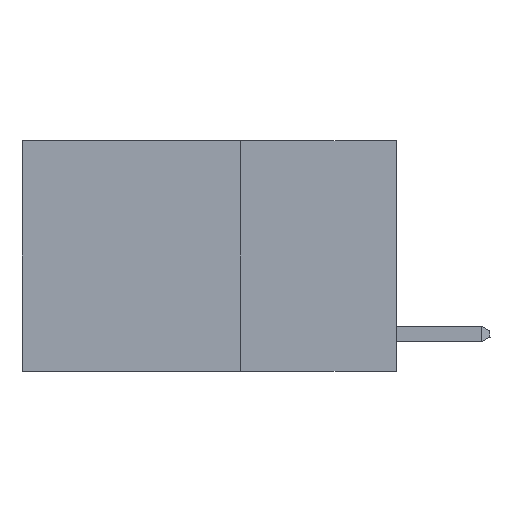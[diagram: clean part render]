
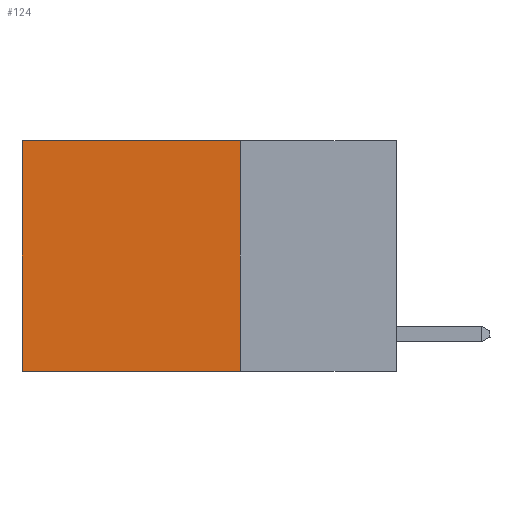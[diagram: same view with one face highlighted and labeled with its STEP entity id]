
A CAD part, left-side view. The second image highlights one B-rep face of the part: STEP entity #124.
In plain terms, the highlighted planar face has unit normal (-1, 0, 0).
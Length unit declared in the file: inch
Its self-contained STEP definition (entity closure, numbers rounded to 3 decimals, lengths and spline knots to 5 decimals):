
#104 = VERTEX_POINT ( 'NONE', #3703 ) ;
#124 = ADVANCED_FACE ( 'NONE', ( #5318 ), #10516, .F. ) ;
#313 = VECTOR ( 'NONE', #4555, 39.37008 ) ;
#640 = EDGE_CURVE ( 'NONE', #3943, #2547, #5304, .T. ) ;
#998 = LINE ( 'NONE', #3549, #4276 ) ;
#1025 = LINE ( 'NONE', #4498, #313 ) ;
#1447 = LINE ( 'NONE', #6322, #2911 ) ;
#1887 = DIRECTION ( 'NONE',  ( 1., 0., 0. ) ) ;
#2547 = VERTEX_POINT ( 'NONE', #10814 ) ;
#2911 = VECTOR ( 'NONE', #7300, 39.37008 ) ;
#3391 = EDGE_LOOP ( 'NONE', ( #7566, #8890, #5827, #5694 ) ) ;
#3517 = VECTOR ( 'NONE', #8070, 39.37008 ) ;
#3549 = CARTESIAN_POINT ( 'NONE',  ( 0.2625, 0.25, 0. ) ) ;
#3703 = CARTESIAN_POINT ( 'NONE',  ( 0.2625, 0.6, -0.37 ) ) ;
#3943 = VERTEX_POINT ( 'NONE', #5110 ) ;
#4020 = EDGE_CURVE ( 'NONE', #2547, #104, #1447, .T. ) ;
#4259 = EDGE_CURVE ( 'NONE', #10767, #104, #1025, .T. ) ;
#4276 = VECTOR ( 'NONE', #7053, 39.37008 ) ;
#4498 = CARTESIAN_POINT ( 'NONE',  ( 0.2625, 0.6, 0. ) ) ;
#4555 = DIRECTION ( 'NONE',  ( 0., 0., -1. ) ) ;
#4563 = CARTESIAN_POINT ( 'NONE',  ( 0.2625, 0.25, 0. ) ) ;
#5110 = CARTESIAN_POINT ( 'NONE',  ( 0.2625, 0.25, 0. ) ) ;
#5304 = LINE ( 'NONE', #4563, #3517 ) ;
#5318 = FACE_OUTER_BOUND ( 'NONE', #3391, .T. ) ;
#5694 = ORIENTED_EDGE ( 'NONE', *, *, #8404, .T. ) ;
#5827 = ORIENTED_EDGE ( 'NONE', *, *, #640, .F. ) ;
#6322 = CARTESIAN_POINT ( 'NONE',  ( 0.2625, 0.25, -0.37 ) ) ;
#7053 = DIRECTION ( 'NONE',  ( 0., 1., 0. ) ) ;
#7155 = DIRECTION ( 'NONE',  ( 0., 0., -1. ) ) ;
#7300 = DIRECTION ( 'NONE',  ( 0., 1., 0. ) ) ;
#7359 = AXIS2_PLACEMENT_3D ( 'NONE', #10686, #1887, #7155 ) ;
#7566 = ORIENTED_EDGE ( 'NONE', *, *, #4259, .T. ) ;
#8070 = DIRECTION ( 'NONE',  ( 0., 0., -1. ) ) ;
#8404 = EDGE_CURVE ( 'NONE', #3943, #10767, #998, .T. ) ;
#8890 = ORIENTED_EDGE ( 'NONE', *, *, #4020, .F. ) ;
#10315 = CARTESIAN_POINT ( 'NONE',  ( 0.2625, 0.6, 0. ) ) ;
#10516 = PLANE ( 'NONE',  #7359 ) ;
#10686 = CARTESIAN_POINT ( 'NONE',  ( 0.2625, 0.25, 0. ) ) ;
#10767 = VERTEX_POINT ( 'NONE', #10315 ) ;
#10814 = CARTESIAN_POINT ( 'NONE',  ( 0.2625, 0.25, -0.37 ) ) ;
